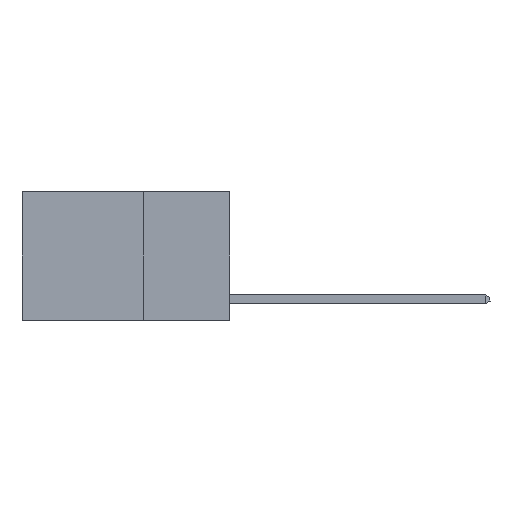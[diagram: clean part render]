
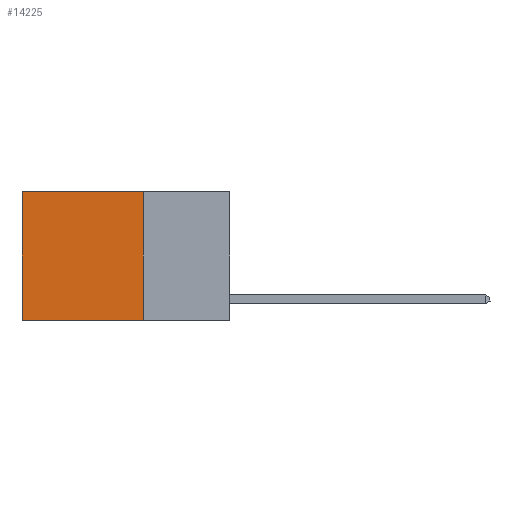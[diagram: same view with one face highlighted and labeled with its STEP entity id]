
A CAD part, left-side view. The second image highlights one B-rep face of the part: STEP entity #14225.
In plain terms, the highlighted planar face has unit normal (-1, 0, 0).
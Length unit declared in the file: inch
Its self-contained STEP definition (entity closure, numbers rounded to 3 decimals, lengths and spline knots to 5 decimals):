
#588 = VERTEX_POINT ( 'NONE', #12187 ) ;
#784 = EDGE_CURVE ( 'NONE', #588, #4766, #12255, .T. ) ;
#804 = CARTESIAN_POINT ( 'NONE',  ( 0.2625, 0.25, 0. ) ) ;
#1002 = DIRECTION ( 'NONE',  ( 0., 0., -1. ) ) ;
#1623 = VECTOR ( 'NONE', #1002, 39.37008 ) ;
#2121 = VECTOR ( 'NONE', #11654, 39.37008 ) ;
#2266 = CARTESIAN_POINT ( 'NONE',  ( 0.2625, 0.6, 0. ) ) ;
#2618 = CARTESIAN_POINT ( 'NONE',  ( 0.2625, 0.25, -0.37 ) ) ;
#3383 = VERTEX_POINT ( 'NONE', #4248 ) ;
#4041 = CARTESIAN_POINT ( 'NONE',  ( 0.2625, 0.6, 0. ) ) ;
#4248 = CARTESIAN_POINT ( 'NONE',  ( 0.2625, 0.6, -0.37 ) ) ;
#4626 = AXIS2_PLACEMENT_3D ( 'NONE', #804, #4806, #13964 ) ;
#4766 = VERTEX_POINT ( 'NONE', #2266 ) ;
#4806 = DIRECTION ( 'NONE',  ( 1., 0., 0. ) ) ;
#6380 = LINE ( 'NONE', #7692, #9482 ) ;
#7692 = CARTESIAN_POINT ( 'NONE',  ( 0.2625, 0.25, -0.37 ) ) ;
#8462 = EDGE_CURVE ( 'NONE', #4766, #3383, #9964, .T. ) ;
#8764 = FACE_OUTER_BOUND ( 'NONE', #9813, .T. ) ;
#9363 = DIRECTION ( 'NONE',  ( 0., 0., -1. ) ) ;
#9482 = VECTOR ( 'NONE', #15375, 39.37008 ) ;
#9813 = EDGE_LOOP ( 'NONE', ( #12108, #12673, #12433, #16083 ) ) ;
#9964 = LINE ( 'NONE', #4041, #16693 ) ;
#10138 = CARTESIAN_POINT ( 'NONE',  ( 0.2625, 0.25, 0. ) ) ;
#11654 = DIRECTION ( 'NONE',  ( 0., 1., 0. ) ) ;
#11743 = EDGE_CURVE ( 'NONE', #15724, #3383, #6380, .T. ) ;
#12108 = ORIENTED_EDGE ( 'NONE', *, *, #8462, .T. ) ;
#12176 = LINE ( 'NONE', #16602, #1623 ) ;
#12187 = CARTESIAN_POINT ( 'NONE',  ( 0.2625, 0.25, 0. ) ) ;
#12255 = LINE ( 'NONE', #10138, #2121 ) ;
#12433 = ORIENTED_EDGE ( 'NONE', *, *, #15590, .F. ) ;
#12673 = ORIENTED_EDGE ( 'NONE', *, *, #11743, .F. ) ;
#12717 = PLANE ( 'NONE',  #4626 ) ;
#13964 = DIRECTION ( 'NONE',  ( 0., 0., -1. ) ) ;
#14225 = ADVANCED_FACE ( 'NONE', ( #8764 ), #12717, .F. ) ;
#15375 = DIRECTION ( 'NONE',  ( 0., 1., 0. ) ) ;
#15590 = EDGE_CURVE ( 'NONE', #588, #15724, #12176, .T. ) ;
#15724 = VERTEX_POINT ( 'NONE', #2618 ) ;
#16083 = ORIENTED_EDGE ( 'NONE', *, *, #784, .T. ) ;
#16602 = CARTESIAN_POINT ( 'NONE',  ( 0.2625, 0.25, 0. ) ) ;
#16693 = VECTOR ( 'NONE', #9363, 39.37008 ) ;
